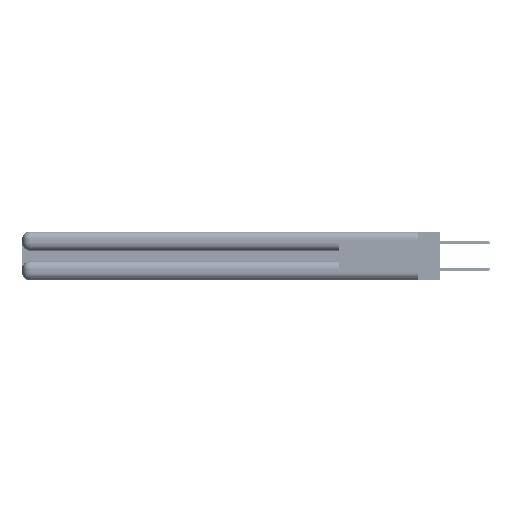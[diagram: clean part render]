
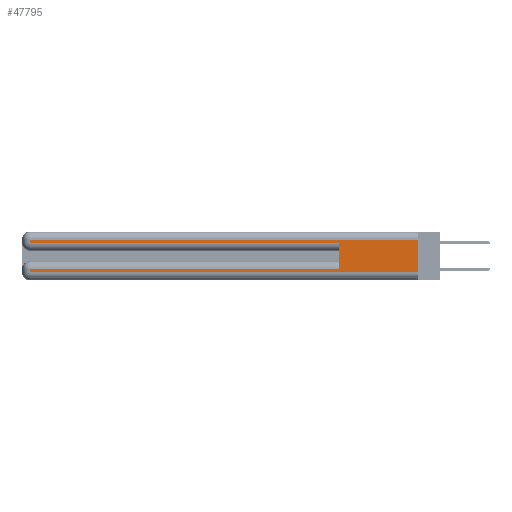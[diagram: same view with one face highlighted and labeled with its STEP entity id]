
A CAD part, left-side view. The second image highlights one B-rep face of the part: STEP entity #47795.
In plain terms, the highlighted planar face has unit normal (-1, 0, 0).
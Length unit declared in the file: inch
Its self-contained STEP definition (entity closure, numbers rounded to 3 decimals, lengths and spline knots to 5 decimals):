
#794 = FACE_OUTER_BOUND ( 'NONE', #3318, .T. ) ;
#973 = VECTOR ( 'NONE', #19887, 39.37008 ) ;
#1661 = VECTOR ( 'NONE', #3792, 39.37008 ) ;
#1882 = CARTESIAN_POINT ( 'NONE',  ( 0., 0.6, 0.285 ) ) ;
#3318 = EDGE_LOOP ( 'NONE', ( #31704, #38927, #18368, #16622, #12794, #47906, #11213, #34317 ) ) ;
#3792 = DIRECTION ( 'NONE',  ( 0., 0., 1. ) ) ;
#4920 = VECTOR ( 'NONE', #45297, 39.37008 ) ;
#7016 = LINE ( 'NONE', #17913, #52370 ) ;
#7483 = AXIS2_PLACEMENT_3D ( 'NONE', #35295, #18296, #48123 ) ;
#8481 = CARTESIAN_POINT ( 'NONE',  ( 0., 2.94, 0.37 ) ) ;
#9223 = EDGE_CURVE ( 'NONE', #39268, #24365, #7016, .T. ) ;
#9669 = LINE ( 'NONE', #22641, #52359 ) ;
#10201 = EDGE_CURVE ( 'NONE', #28029, #38728, #35007, .T. ) ;
#10881 = LINE ( 'NONE', #8481, #54861 ) ;
#11185 = CARTESIAN_POINT ( 'NONE',  ( 0., 2.94, 0.37 ) ) ;
#11213 = ORIENTED_EDGE ( 'NONE', *, *, #40756, .T. ) ;
#12794 = ORIENTED_EDGE ( 'NONE', *, *, #40168, .F. ) ;
#13402 = EDGE_CURVE ( 'NONE', #19281, #22082, #40726, .T. ) ;
#16054 = CARTESIAN_POINT ( 'NONE',  ( 0., 0., 0.06 ) ) ;
#16622 = ORIENTED_EDGE ( 'NONE', *, *, #10201, .T. ) ;
#17051 = DIRECTION ( 'NONE',  ( 0., 0., -1. ) ) ;
#17913 = CARTESIAN_POINT ( 'NONE',  ( 0., 0., 0.085 ) ) ;
#18296 = DIRECTION ( 'NONE',  ( 1., 0., 0. ) ) ;
#18368 = ORIENTED_EDGE ( 'NONE', *, *, #53594, .T. ) ;
#18514 = VERTEX_POINT ( 'NONE', #33341 ) ;
#19281 = VERTEX_POINT ( 'NONE', #31033 ) ;
#19887 = DIRECTION ( 'NONE',  ( 0., -1., 0. ) ) ;
#20695 = CARTESIAN_POINT ( 'NONE',  ( 0., 2.94, 0.085 ) ) ;
#22082 = VERTEX_POINT ( 'NONE', #16054 ) ;
#22641 = CARTESIAN_POINT ( 'NONE',  ( 0., 0., 0.31 ) ) ;
#24365 = VERTEX_POINT ( 'NONE', #20695 ) ;
#25491 = EDGE_CURVE ( 'NONE', #36533, #22082, #53007, .T. ) ;
#28029 = VERTEX_POINT ( 'NONE', #37212 ) ;
#28208 = CARTESIAN_POINT ( 'NONE',  ( 0., 0., 0.37 ) ) ;
#30348 = VECTOR ( 'NONE', #53748, 39.37008 ) ;
#31033 = CARTESIAN_POINT ( 'NONE',  ( 0., 2.94, 0.06 ) ) ;
#31704 = ORIENTED_EDGE ( 'NONE', *, *, #25491, .F. ) ;
#33341 = CARTESIAN_POINT ( 'NONE',  ( 0., 2.94, 0.31 ) ) ;
#34317 = ORIENTED_EDGE ( 'NONE', *, *, #13402, .T. ) ;
#35007 = LINE ( 'NONE', #49687, #973 ) ;
#35295 = CARTESIAN_POINT ( 'NONE',  ( 0., 0., 0.37 ) ) ;
#35698 = LINE ( 'NONE', #54807, #1661 ) ;
#36533 = VERTEX_POINT ( 'NONE', #53364 ) ;
#37212 = CARTESIAN_POINT ( 'NONE',  ( 0., 2.94, 0.285 ) ) ;
#38013 = CARTESIAN_POINT ( 'NONE',  ( 0., 0., 0.06 ) ) ;
#38728 = VERTEX_POINT ( 'NONE', #1882 ) ;
#38927 = ORIENTED_EDGE ( 'NONE', *, *, #45300, .T. ) ;
#39268 = VERTEX_POINT ( 'NONE', #39867 ) ;
#39361 = DIRECTION ( 'NONE',  ( 0., 1., 0. ) ) ;
#39560 = PLANE ( 'NONE',  #7483 ) ;
#39867 = CARTESIAN_POINT ( 'NONE',  ( 0., 0.6, 0.085 ) ) ;
#40168 = EDGE_CURVE ( 'NONE', #39268, #38728, #35698, .T. ) ;
#40726 = LINE ( 'NONE', #38013, #42083 ) ;
#40756 = EDGE_CURVE ( 'NONE', #24365, #19281, #50248, .T. ) ;
#42083 = VECTOR ( 'NONE', #46612, 39.37008 ) ;
#45297 = DIRECTION ( 'NONE',  ( 0., 0., -1. ) ) ;
#45300 = EDGE_CURVE ( 'NONE', #36533, #18514, #9669, .T. ) ;
#46612 = DIRECTION ( 'NONE',  ( 0., -1., 0. ) ) ;
#47795 = ADVANCED_FACE ( 'NONE', ( #794 ), #39560, .F. ) ;
#47906 = ORIENTED_EDGE ( 'NONE', *, *, #9223, .T. ) ;
#48123 = DIRECTION ( 'NONE',  ( 0., 0., -1. ) ) ;
#49687 = CARTESIAN_POINT ( 'NONE',  ( 0., 0., 0.285 ) ) ;
#50248 = LINE ( 'NONE', #11185, #4920 ) ;
#52359 = VECTOR ( 'NONE', #52485, 39.37008 ) ;
#52370 = VECTOR ( 'NONE', #39361, 39.37008 ) ;
#52485 = DIRECTION ( 'NONE',  ( 0., 1., 0. ) ) ;
#53007 = LINE ( 'NONE', #28208, #30348 ) ;
#53364 = CARTESIAN_POINT ( 'NONE',  ( 0., 0., 0.31 ) ) ;
#53594 = EDGE_CURVE ( 'NONE', #18514, #28029, #10881, .T. ) ;
#53748 = DIRECTION ( 'NONE',  ( 0., 0., -1. ) ) ;
#54807 = CARTESIAN_POINT ( 'NONE',  ( 0., 0.6, 0.145 ) ) ;
#54861 = VECTOR ( 'NONE', #17051, 39.37008 ) ;
